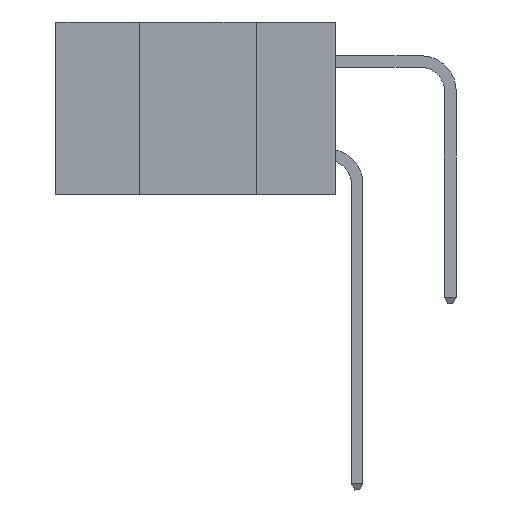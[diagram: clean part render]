
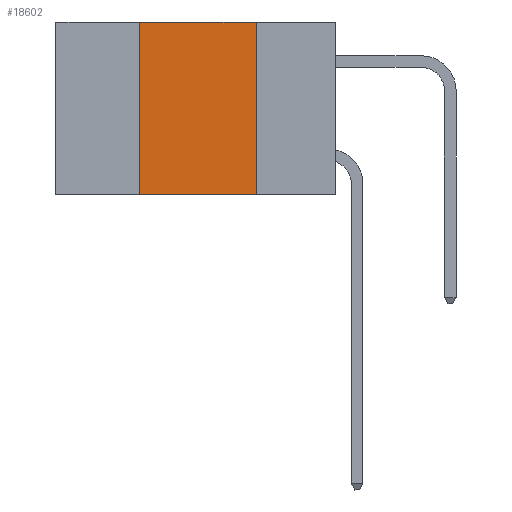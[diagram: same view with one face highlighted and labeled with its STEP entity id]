
A CAD part, left-side view. The second image highlights one B-rep face of the part: STEP entity #18602.
In plain terms, the highlighted planar face has unit normal (-1, 0, 0).
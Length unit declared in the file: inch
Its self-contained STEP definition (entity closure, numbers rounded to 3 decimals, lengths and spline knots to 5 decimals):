
#261 = FACE_OUTER_BOUND ( 'NONE', #8992, .T. ) ;
#1059 = CARTESIAN_POINT ( 'NONE',  ( 0., 0.6, -0.37 ) ) ;
#2852 = PLANE ( 'NONE',  #12474 ) ;
#3468 = VECTOR ( 'NONE', #18322, 39.37008 ) ;
#4901 = DIRECTION ( 'NONE',  ( 0., 0., 1. ) ) ;
#5220 = LINE ( 'NONE', #27044, #6920 ) ;
#5289 = DIRECTION ( 'NONE',  ( 1., 0., 0. ) ) ;
#5607 = VECTOR ( 'NONE', #22032, 39.37008 ) ;
#6046 = LINE ( 'NONE', #23029, #3468 ) ;
#6920 = VECTOR ( 'NONE', #4901, 39.37008 ) ;
#6935 = VERTEX_POINT ( 'NONE', #18277 ) ;
#7743 = VERTEX_POINT ( 'NONE', #9831 ) ;
#8992 = EDGE_LOOP ( 'NONE', ( #18334, #23894, #12094, #21151 ) ) ;
#9831 = CARTESIAN_POINT ( 'NONE',  ( 0., 0.42, -0.37 ) ) ;
#12094 = ORIENTED_EDGE ( 'NONE', *, *, #22601, .F. ) ;
#12338 = LINE ( 'NONE', #24619, #5607 ) ;
#12474 = AXIS2_PLACEMENT_3D ( 'NONE', #29837, #5289, #25006 ) ;
#14216 = CARTESIAN_POINT ( 'NONE',  ( 0., 0.17, -0.37 ) ) ;
#15780 = LINE ( 'NONE', #1059, #29019 ) ;
#18277 = CARTESIAN_POINT ( 'NONE',  ( 0., 0.42, 0. ) ) ;
#18322 = DIRECTION ( 'NONE',  ( 0., -1., 0. ) ) ;
#18334 = ORIENTED_EDGE ( 'NONE', *, *, #28143, .F. ) ;
#18602 = ADVANCED_FACE ( 'NONE', ( #261 ), #2852, .F. ) ;
#18640 = EDGE_CURVE ( 'NONE', #7743, #30393, #15780, .T. ) ;
#19323 = CARTESIAN_POINT ( 'NONE',  ( 0., 0.17, 0. ) ) ;
#21151 = ORIENTED_EDGE ( 'NONE', *, *, #18640, .T. ) ;
#22032 = DIRECTION ( 'NONE',  ( 0., 0., -1. ) ) ;
#22601 = EDGE_CURVE ( 'NONE', #7743, #6935, #5220, .T. ) ;
#23029 = CARTESIAN_POINT ( 'NONE',  ( 0., 0.6, 0. ) ) ;
#23894 = ORIENTED_EDGE ( 'NONE', *, *, #26503, .F. ) ;
#24619 = CARTESIAN_POINT ( 'NONE',  ( 0., 0.17, 0. ) ) ;
#25006 = DIRECTION ( 'NONE',  ( 0., 0., -1. ) ) ;
#25162 = DIRECTION ( 'NONE',  ( 0., -1., 0. ) ) ;
#26503 = EDGE_CURVE ( 'NONE', #6935, #27763, #6046, .T. ) ;
#27044 = CARTESIAN_POINT ( 'NONE',  ( 0., 0.42, 0. ) ) ;
#27763 = VERTEX_POINT ( 'NONE', #19323 ) ;
#28143 = EDGE_CURVE ( 'NONE', #27763, #30393, #12338, .T. ) ;
#29019 = VECTOR ( 'NONE', #25162, 39.37008 ) ;
#29837 = CARTESIAN_POINT ( 'NONE',  ( 0., 0.6, 0. ) ) ;
#30393 = VERTEX_POINT ( 'NONE', #14216 ) ;
